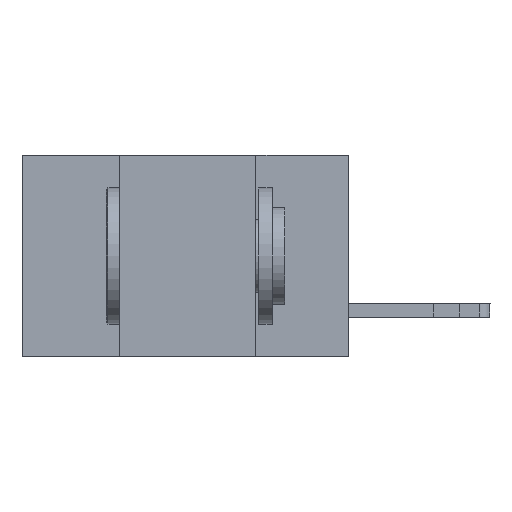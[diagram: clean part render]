
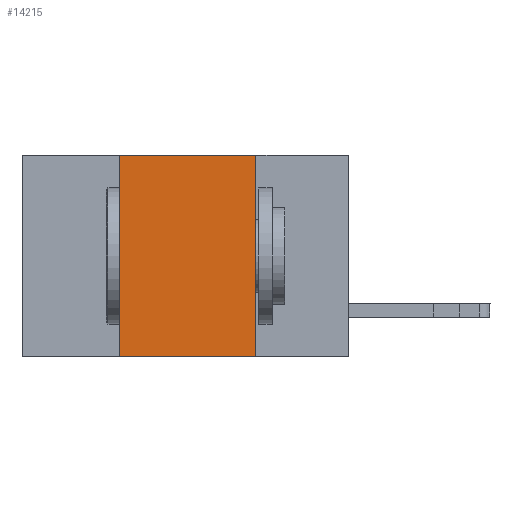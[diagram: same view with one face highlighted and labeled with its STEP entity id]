
A CAD part, left-side view. The second image highlights one B-rep face of the part: STEP entity #14215.
In plain terms, the highlighted planar face has unit normal (-1, 0, 0).
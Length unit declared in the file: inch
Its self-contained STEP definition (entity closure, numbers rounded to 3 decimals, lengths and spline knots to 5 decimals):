
#1309 = LINE ( 'NONE', #8081, #5784 ) ;
#3752 = LINE ( 'NONE', #24041, #19431 ) ;
#4320 = DIRECTION ( 'NONE',  ( 1., 0., 0. ) ) ;
#5263 = VECTOR ( 'NONE', #13095, 39.37008 ) ;
#5784 = VECTOR ( 'NONE', #14337, 39.37008 ) ;
#5986 = CARTESIAN_POINT ( 'NONE',  ( 0., 0.6, 0. ) ) ;
#6403 = EDGE_CURVE ( 'NONE', #11444, #18245, #1309, .T. ) ;
#6449 = CARTESIAN_POINT ( 'NONE',  ( 0., 0.42, 0. ) ) ;
#7063 = VECTOR ( 'NONE', #22289, 39.37008 ) ;
#8081 = CARTESIAN_POINT ( 'NONE',  ( 0., 0.42, 0. ) ) ;
#8427 = EDGE_CURVE ( 'NONE', #10404, #16522, #3752, .T. ) ;
#8702 = CARTESIAN_POINT ( 'NONE',  ( 0., 0.17, 0. ) ) ;
#8823 = EDGE_LOOP ( 'NONE', ( #23091, #17440, #16705, #19690 ) ) ;
#9617 = DIRECTION ( 'NONE',  ( 0., 0., -1. ) ) ;
#10404 = VERTEX_POINT ( 'NONE', #8702 ) ;
#10423 = CARTESIAN_POINT ( 'NONE',  ( 0., 0.6, -0.37 ) ) ;
#11444 = VERTEX_POINT ( 'NONE', #21440 ) ;
#11453 = FACE_OUTER_BOUND ( 'NONE', #8823, .T. ) ;
#11817 = LINE ( 'NONE', #5986, #7063 ) ;
#13095 = DIRECTION ( 'NONE',  ( 0., -1., 0. ) ) ;
#14215 = ADVANCED_FACE ( 'NONE', ( #11453 ), #22771, .F. ) ;
#14337 = DIRECTION ( 'NONE',  ( 0., 0., 1. ) ) ;
#15426 = EDGE_CURVE ( 'NONE', #11444, #16522, #19351, .T. ) ;
#15475 = AXIS2_PLACEMENT_3D ( 'NONE', #22139, #4320, #16566 ) ;
#16522 = VERTEX_POINT ( 'NONE', #19268 ) ;
#16566 = DIRECTION ( 'NONE',  ( 0., 0., -1. ) ) ;
#16705 = ORIENTED_EDGE ( 'NONE', *, *, #6403, .F. ) ;
#17440 = ORIENTED_EDGE ( 'NONE', *, *, #23010, .F. ) ;
#18245 = VERTEX_POINT ( 'NONE', #6449 ) ;
#19268 = CARTESIAN_POINT ( 'NONE',  ( 0., 0.17, -0.37 ) ) ;
#19351 = LINE ( 'NONE', #10423, #5263 ) ;
#19431 = VECTOR ( 'NONE', #9617, 39.37008 ) ;
#19690 = ORIENTED_EDGE ( 'NONE', *, *, #15426, .T. ) ;
#21440 = CARTESIAN_POINT ( 'NONE',  ( 0., 0.42, -0.37 ) ) ;
#22139 = CARTESIAN_POINT ( 'NONE',  ( 0., 0.6, 0. ) ) ;
#22289 = DIRECTION ( 'NONE',  ( 0., -1., 0. ) ) ;
#22771 = PLANE ( 'NONE',  #15475 ) ;
#23010 = EDGE_CURVE ( 'NONE', #18245, #10404, #11817, .T. ) ;
#23091 = ORIENTED_EDGE ( 'NONE', *, *, #8427, .F. ) ;
#24041 = CARTESIAN_POINT ( 'NONE',  ( 0., 0.17, 0. ) ) ;
